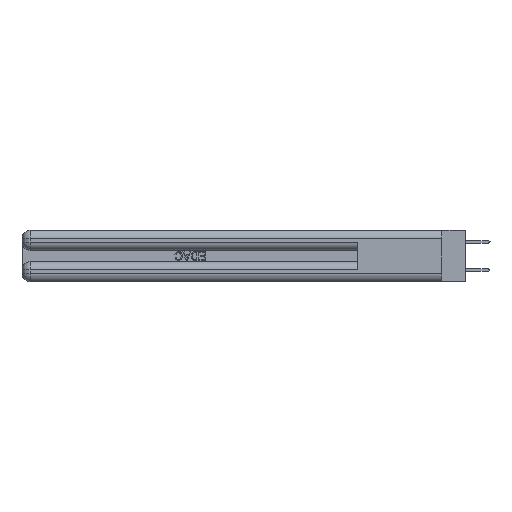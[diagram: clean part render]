
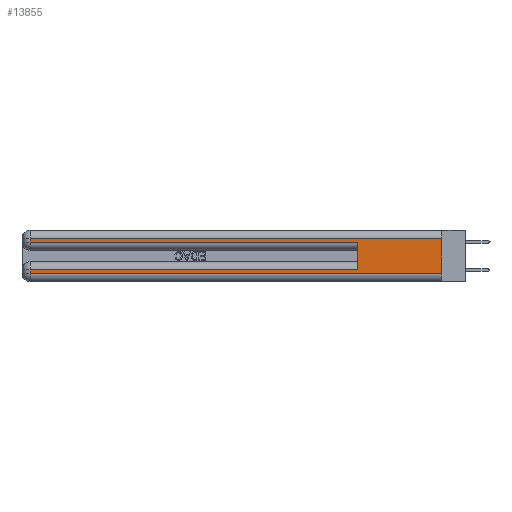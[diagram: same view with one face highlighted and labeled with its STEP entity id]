
A CAD part, left-side view. The second image highlights one B-rep face of the part: STEP entity #13855.
In plain terms, the highlighted planar face has unit normal (-1, 0, 0).
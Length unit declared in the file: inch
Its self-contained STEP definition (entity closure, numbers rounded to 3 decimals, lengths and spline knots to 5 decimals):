
#39 = DIRECTION ( 'NONE',  ( 1., 0., 0. ) ) ;
#314 = ORIENTED_EDGE ( 'NONE', *, *, #2336, .T. ) ;
#692 = VERTEX_POINT ( 'NONE', #4604 ) ;
#1588 = VERTEX_POINT ( 'NONE', #33240 ) ;
#2336 = EDGE_CURVE ( 'NONE', #692, #24684, #6638, .T. ) ;
#2349 = EDGE_LOOP ( 'NONE', ( #40277, #16814, #4448, #3370, #10896, #10915, #38286, #314 ) ) ;
#3370 = ORIENTED_EDGE ( 'NONE', *, *, #35249, .T. ) ;
#3732 = VECTOR ( 'NONE', #25352, 39.37008 ) ;
#3937 = CARTESIAN_POINT ( 'NONE',  ( 0., 0., 0.37 ) ) ;
#4002 = CARTESIAN_POINT ( 'NONE',  ( 0., 0., 0.06 ) ) ;
#4144 = DIRECTION ( 'NONE',  ( 0., -1., 0. ) ) ;
#4448 = ORIENTED_EDGE ( 'NONE', *, *, #27347, .T. ) ;
#4604 = CARTESIAN_POINT ( 'NONE',  ( 0., 2.94, 0.06 ) ) ;
#5126 = VECTOR ( 'NONE', #28830, 39.37008 ) ;
#5286 = LINE ( 'NONE', #34545, #22645 ) ;
#6638 = LINE ( 'NONE', #4002, #40247 ) ;
#7706 = VECTOR ( 'NONE', #9766, 39.37008 ) ;
#8107 = EDGE_CURVE ( 'NONE', #1588, #23405, #13462, .T. ) ;
#9438 = DIRECTION ( 'NONE',  ( 0., 0., -1. ) ) ;
#9766 = DIRECTION ( 'NONE',  ( 0., 0., 1. ) ) ;
#10896 = ORIENTED_EDGE ( 'NONE', *, *, #35800, .F. ) ;
#10915 = ORIENTED_EDGE ( 'NONE', *, *, #8107, .T. ) ;
#12418 = CARTESIAN_POINT ( 'NONE',  ( 0., 0., 0.085 ) ) ;
#12652 = CARTESIAN_POINT ( 'NONE',  ( 0., 0., 0.285 ) ) ;
#13462 = LINE ( 'NONE', #12418, #3732 ) ;
#13855 = ADVANCED_FACE ( 'NONE', ( #41875 ), #39196, .F. ) ;
#16442 = CARTESIAN_POINT ( 'NONE',  ( 0., 0., 0.37 ) ) ;
#16801 = AXIS2_PLACEMENT_3D ( 'NONE', #16442, #39, #22998 ) ;
#16814 = ORIENTED_EDGE ( 'NONE', *, *, #32680, .T. ) ;
#18653 = CARTESIAN_POINT ( 'NONE',  ( 0., 0.6, 0.285 ) ) ;
#19453 = VECTOR ( 'NONE', #24273, 39.37008 ) ;
#20891 = CARTESIAN_POINT ( 'NONE',  ( 0., 2.94, 0.37 ) ) ;
#22645 = VECTOR ( 'NONE', #28030, 39.37008 ) ;
#22877 = CARTESIAN_POINT ( 'NONE',  ( 0., 2.94, 0.285 ) ) ;
#22998 = DIRECTION ( 'NONE',  ( 0., 0., -1. ) ) ;
#23405 = VERTEX_POINT ( 'NONE', #34144 ) ;
#23691 = EDGE_CURVE ( 'NONE', #23405, #692, #36472, .T. ) ;
#23992 = LINE ( 'NONE', #39050, #7706 ) ;
#24273 = DIRECTION ( 'NONE',  ( 0., 0., -1. ) ) ;
#24684 = VERTEX_POINT ( 'NONE', #40561 ) ;
#24773 = CARTESIAN_POINT ( 'NONE',  ( 0., 2.94, 0.31 ) ) ;
#25352 = DIRECTION ( 'NONE',  ( 0., 1., 0. ) ) ;
#26739 = DIRECTION ( 'NONE',  ( 0., 0., -1. ) ) ;
#27347 = EDGE_CURVE ( 'NONE', #38063, #31686, #38768, .T. ) ;
#28030 = DIRECTION ( 'NONE',  ( 0., 1., 0. ) ) ;
#28830 = DIRECTION ( 'NONE',  ( 0., -1., 0. ) ) ;
#28836 = VECTOR ( 'NONE', #9438, 39.37008 ) ;
#28980 = VERTEX_POINT ( 'NONE', #18653 ) ;
#29716 = LINE ( 'NONE', #3937, #38362 ) ;
#30331 = CARTESIAN_POINT ( 'NONE',  ( 0., 0., 0.31 ) ) ;
#30516 = VERTEX_POINT ( 'NONE', #30331 ) ;
#31102 = LINE ( 'NONE', #12652, #5126 ) ;
#31686 = VERTEX_POINT ( 'NONE', #22877 ) ;
#32303 = CARTESIAN_POINT ( 'NONE',  ( 0., 2.94, 0.37 ) ) ;
#32680 = EDGE_CURVE ( 'NONE', #30516, #38063, #5286, .T. ) ;
#32920 = EDGE_CURVE ( 'NONE', #30516, #24684, #29716, .T. ) ;
#33240 = CARTESIAN_POINT ( 'NONE',  ( 0., 0.6, 0.085 ) ) ;
#34144 = CARTESIAN_POINT ( 'NONE',  ( 0., 2.94, 0.085 ) ) ;
#34545 = CARTESIAN_POINT ( 'NONE',  ( 0., 0., 0.31 ) ) ;
#35249 = EDGE_CURVE ( 'NONE', #31686, #28980, #31102, .T. ) ;
#35800 = EDGE_CURVE ( 'NONE', #1588, #28980, #23992, .T. ) ;
#36472 = LINE ( 'NONE', #32303, #28836 ) ;
#38063 = VERTEX_POINT ( 'NONE', #24773 ) ;
#38286 = ORIENTED_EDGE ( 'NONE', *, *, #23691, .T. ) ;
#38362 = VECTOR ( 'NONE', #26739, 39.37008 ) ;
#38768 = LINE ( 'NONE', #20891, #19453 ) ;
#39050 = CARTESIAN_POINT ( 'NONE',  ( 0., 0.6, 0.145 ) ) ;
#39196 = PLANE ( 'NONE',  #16801 ) ;
#40247 = VECTOR ( 'NONE', #4144, 39.37008 ) ;
#40277 = ORIENTED_EDGE ( 'NONE', *, *, #32920, .F. ) ;
#40561 = CARTESIAN_POINT ( 'NONE',  ( 0., 0., 0.06 ) ) ;
#41875 = FACE_OUTER_BOUND ( 'NONE', #2349, .T. ) ;
